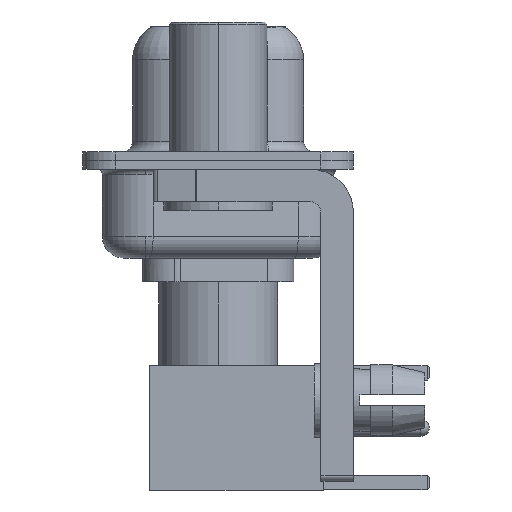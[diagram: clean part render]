
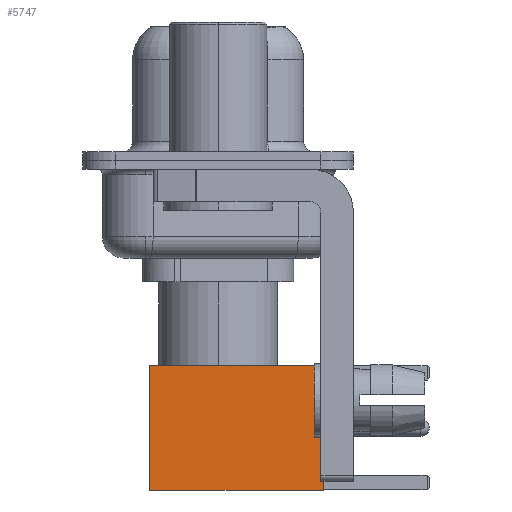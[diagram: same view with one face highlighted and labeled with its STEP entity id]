
A CAD part, left-side view. The second image highlights one B-rep face of the part: STEP entity #5747.
In plain terms, the highlighted face is planar.
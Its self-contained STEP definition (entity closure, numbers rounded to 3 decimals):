
#33 = CARTESIAN_POINT ( 'NONE',  ( 2.875, 2.875, 0. ) ) ;
#772 = VERTEX_POINT ( 'NONE', #33 ) ;
#1487 = EDGE_CURVE ( 'NONE', #772, #12996, #8339, .T. ) ;
#1837 = CARTESIAN_POINT ( 'NONE',  ( -2.875, 2.875, 0. ) ) ;
#2659 = ORIENTED_EDGE ( 'NONE', *, *, #18908, .F. ) ;
#3383 = CARTESIAN_POINT ( 'NONE',  ( 0., 2.875, 0. ) ) ;
#3598 = CARTESIAN_POINT ( 'NONE',  ( -2.875, 2.875, 0. ) ) ;
#3966 = VECTOR ( 'NONE', #18884, 1000. ) ;
#4023 = VECTOR ( 'NONE', #6969, 1000. ) ;
#4612 = EDGE_CURVE ( 'NONE', #18863, #772, #17759, .T. ) ;
#4881 = ORIENTED_EDGE ( 'NONE', *, *, #4612, .T. ) ;
#4985 = LINE ( 'NONE', #3598, #4023 ) ;
#5375 = PLANE ( 'NONE',  #13330 ) ;
#5671 = CARTESIAN_POINT ( 'NONE',  ( 2.875, 2.875, 0. ) ) ;
#5679 = ORIENTED_EDGE ( 'NONE', *, *, #16701, .F. ) ;
#5747 = ADVANCED_FACE ( 'NONE', ( #13164 ), #5375, .T. ) ;
#6353 = CARTESIAN_POINT ( 'NONE',  ( -2.875, 2.875, 8. ) ) ;
#6816 = CARTESIAN_POINT ( 'NONE',  ( 0., 2.875, 8. ) ) ;
#6969 = DIRECTION ( 'NONE',  ( 0., 0., -1. ) ) ;
#7562 = DIRECTION ( 'NONE',  ( 0., 0., -1. ) ) ;
#8051 = EDGE_LOOP ( 'NONE', ( #4881, #8663, #2659, #5679 ) ) ;
#8339 = LINE ( 'NONE', #3383, #12028 ) ;
#8663 = ORIENTED_EDGE ( 'NONE', *, *, #1487, .T. ) ;
#10215 = CARTESIAN_POINT ( 'NONE',  ( 2.875, 2.875, 0. ) ) ;
#11315 = DIRECTION ( 'NONE',  ( 0., 1., 0. ) ) ;
#12028 = VECTOR ( 'NONE', #12864, 1000. ) ;
#12864 = DIRECTION ( 'NONE',  ( -1., 0., 0. ) ) ;
#12996 = VERTEX_POINT ( 'NONE', #1837 ) ;
#13164 = FACE_OUTER_BOUND ( 'NONE', #8051, .T. ) ;
#13330 = AXIS2_PLACEMENT_3D ( 'NONE', #5671, #11315, #14645 ) ;
#14259 = CARTESIAN_POINT ( 'NONE',  ( 2.875, 2.875, 8. ) ) ;
#14577 = VECTOR ( 'NONE', #7562, 1000. ) ;
#14645 = DIRECTION ( 'NONE',  ( 0., 0., 1. ) ) ;
#15893 = LINE ( 'NONE', #6816, #3966 ) ;
#16701 = EDGE_CURVE ( 'NONE', #18863, #19215, #15893, .T. ) ;
#17759 = LINE ( 'NONE', #10215, #14577 ) ;
#18863 = VERTEX_POINT ( 'NONE', #14259 ) ;
#18884 = DIRECTION ( 'NONE',  ( -1., 0., 0. ) ) ;
#18908 = EDGE_CURVE ( 'NONE', #19215, #12996, #4985, .T. ) ;
#19215 = VERTEX_POINT ( 'NONE', #6353 ) ;
